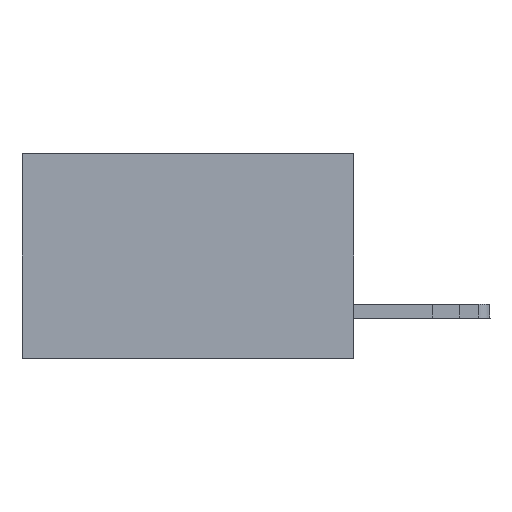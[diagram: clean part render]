
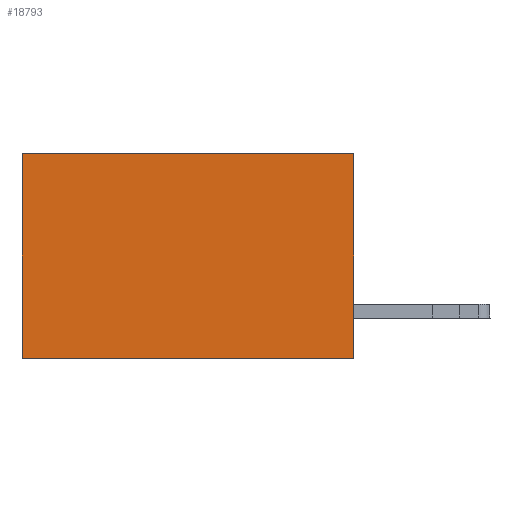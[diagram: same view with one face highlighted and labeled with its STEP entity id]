
A CAD part, left-side view. The second image highlights one B-rep face of the part: STEP entity #18793.
In plain terms, the highlighted planar face has unit normal (-1, 0, 0).
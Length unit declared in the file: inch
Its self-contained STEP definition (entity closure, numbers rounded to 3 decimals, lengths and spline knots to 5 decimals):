
#509 = EDGE_CURVE ( 'NONE', #3663, #10116, #15595, .T. ) ;
#1005 = EDGE_LOOP ( 'NONE', ( #21346, #15894, #3772, #9819 ) ) ;
#1181 = PLANE ( 'NONE',  #13487 ) ;
#2183 = LINE ( 'NONE', #20299, #12159 ) ;
#2575 = LINE ( 'NONE', #8600, #18523 ) ;
#2702 = CARTESIAN_POINT ( 'NONE',  ( 0.2875, 0., 0. ) ) ;
#3483 = CARTESIAN_POINT ( 'NONE',  ( 0.2875, 0., 0. ) ) ;
#3663 = VERTEX_POINT ( 'NONE', #26095 ) ;
#3772 = ORIENTED_EDGE ( 'NONE', *, *, #18214, .F. ) ;
#7994 = LINE ( 'NONE', #2702, #13053 ) ;
#8600 = CARTESIAN_POINT ( 'NONE',  ( 0.2875, 0.6, 0. ) ) ;
#9819 = ORIENTED_EDGE ( 'NONE', *, *, #509, .T. ) ;
#10116 = VERTEX_POINT ( 'NONE', #15791 ) ;
#10797 = CARTESIAN_POINT ( 'NONE',  ( 0.2875, 0.6, -0.37 ) ) ;
#10959 = FACE_OUTER_BOUND ( 'NONE', #1005, .T. ) ;
#11336 = DIRECTION ( 'NONE',  ( 0., 0., -1. ) ) ;
#11702 = CARTESIAN_POINT ( 'NONE',  ( 0.2875, 0., -0.37 ) ) ;
#12159 = VECTOR ( 'NONE', #22790, 39.37008 ) ;
#12835 = DIRECTION ( 'NONE',  ( 0., 0., -1. ) ) ;
#13053 = VECTOR ( 'NONE', #12835, 39.37008 ) ;
#13487 = AXIS2_PLACEMENT_3D ( 'NONE', #19051, #25557, #11336 ) ;
#14020 = EDGE_CURVE ( 'NONE', #10116, #22500, #2575, .T. ) ;
#15595 = LINE ( 'NONE', #3483, #20284 ) ;
#15791 = CARTESIAN_POINT ( 'NONE',  ( 0.2875, 0.6, 0. ) ) ;
#15894 = ORIENTED_EDGE ( 'NONE', *, *, #16935, .F. ) ;
#16935 = EDGE_CURVE ( 'NONE', #19412, #22500, #2183, .T. ) ;
#18214 = EDGE_CURVE ( 'NONE', #3663, #19412, #7994, .T. ) ;
#18523 = VECTOR ( 'NONE', #21201, 39.37008 ) ;
#18793 = ADVANCED_FACE ( 'NONE', ( #10959 ), #1181, .F. ) ;
#19051 = CARTESIAN_POINT ( 'NONE',  ( 0.2875, 0., 0. ) ) ;
#19412 = VERTEX_POINT ( 'NONE', #11702 ) ;
#20284 = VECTOR ( 'NONE', #22238, 39.37008 ) ;
#20299 = CARTESIAN_POINT ( 'NONE',  ( 0.2875, 0., -0.37 ) ) ;
#21201 = DIRECTION ( 'NONE',  ( 0., 0., -1. ) ) ;
#21346 = ORIENTED_EDGE ( 'NONE', *, *, #14020, .T. ) ;
#22238 = DIRECTION ( 'NONE',  ( 0., 1., 0. ) ) ;
#22500 = VERTEX_POINT ( 'NONE', #10797 ) ;
#22790 = DIRECTION ( 'NONE',  ( 0., 1., 0. ) ) ;
#25557 = DIRECTION ( 'NONE',  ( 1., 0., 0. ) ) ;
#26095 = CARTESIAN_POINT ( 'NONE',  ( 0.2875, 0., 0. ) ) ;
